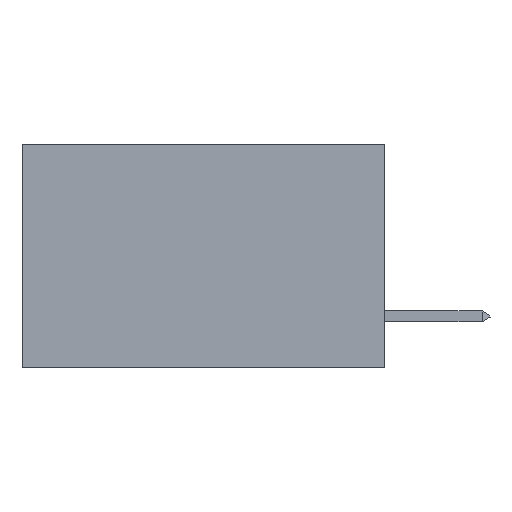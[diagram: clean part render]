
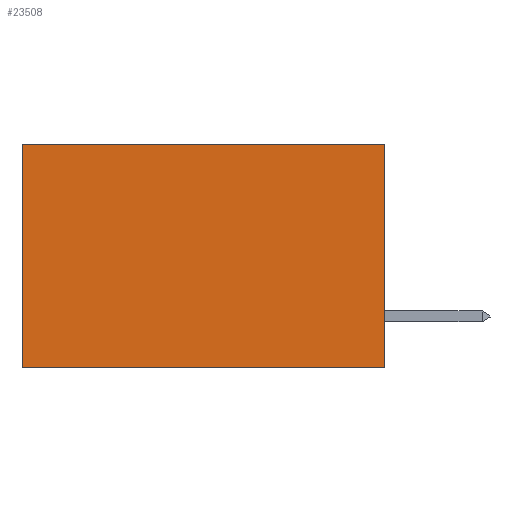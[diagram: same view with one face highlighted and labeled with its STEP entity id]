
A CAD part, left-side view. The second image highlights one B-rep face of the part: STEP entity #23508.
In plain terms, the highlighted planar face has unit normal (-1, 0, 0).
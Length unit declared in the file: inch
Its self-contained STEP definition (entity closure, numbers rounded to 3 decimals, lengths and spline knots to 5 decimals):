
#520 = ORIENTED_EDGE ( 'NONE', *, *, #11956, .F. ) ;
#1276 = EDGE_CURVE ( 'NONE', #7058, #15174, #4210, .T. ) ;
#1391 = ORIENTED_EDGE ( 'NONE', *, *, #22972, .F. ) ;
#1559 = CARTESIAN_POINT ( 'NONE',  ( 0.2875, 0., 0. ) ) ;
#1626 = VECTOR ( 'NONE', #16378, 39.37008 ) ;
#1716 = VECTOR ( 'NONE', #12483, 39.37008 ) ;
#3242 = CARTESIAN_POINT ( 'NONE',  ( 0.2875, 0., 0. ) ) ;
#3278 = DIRECTION ( 'NONE',  ( 0., 1., 0. ) ) ;
#3749 = LINE ( 'NONE', #4835, #1716 ) ;
#4210 = LINE ( 'NONE', #1559, #6255 ) ;
#4835 = CARTESIAN_POINT ( 'NONE',  ( 0.2875, 0.6, 0. ) ) ;
#6255 = VECTOR ( 'NONE', #3278, 39.37008 ) ;
#7043 = AXIS2_PLACEMENT_3D ( 'NONE', #15377, #22719, #13527 ) ;
#7058 = VERTEX_POINT ( 'NONE', #3242 ) ;
#7278 = VERTEX_POINT ( 'NONE', #19413 ) ;
#8296 = ORIENTED_EDGE ( 'NONE', *, *, #1276, .T. ) ;
#10164 = FACE_OUTER_BOUND ( 'NONE', #10364, .T. ) ;
#10183 = EDGE_CURVE ( 'NONE', #15174, #14729, #3749, .T. ) ;
#10364 = EDGE_LOOP ( 'NONE', ( #19242, #1391, #520, #8296 ) ) ;
#10704 = CARTESIAN_POINT ( 'NONE',  ( 0.2875, 0.6, -0.37 ) ) ;
#11956 = EDGE_CURVE ( 'NONE', #7058, #7278, #13223, .T. ) ;
#12483 = DIRECTION ( 'NONE',  ( 0., 0., -1. ) ) ;
#13223 = LINE ( 'NONE', #16225, #1626 ) ;
#13447 = PLANE ( 'NONE',  #7043 ) ;
#13527 = DIRECTION ( 'NONE',  ( 0., 0., -1. ) ) ;
#13793 = DIRECTION ( 'NONE',  ( 0., 1., 0. ) ) ;
#14729 = VERTEX_POINT ( 'NONE', #10704 ) ;
#15174 = VERTEX_POINT ( 'NONE', #18854 ) ;
#15377 = CARTESIAN_POINT ( 'NONE',  ( 0.2875, 0., 0. ) ) ;
#15714 = CARTESIAN_POINT ( 'NONE',  ( 0.2875, 0., -0.37 ) ) ;
#15948 = LINE ( 'NONE', #15714, #23793 ) ;
#16225 = CARTESIAN_POINT ( 'NONE',  ( 0.2875, 0., 0. ) ) ;
#16378 = DIRECTION ( 'NONE',  ( 0., 0., -1. ) ) ;
#18854 = CARTESIAN_POINT ( 'NONE',  ( 0.2875, 0.6, 0. ) ) ;
#19242 = ORIENTED_EDGE ( 'NONE', *, *, #10183, .T. ) ;
#19413 = CARTESIAN_POINT ( 'NONE',  ( 0.2875, 0., -0.37 ) ) ;
#22719 = DIRECTION ( 'NONE',  ( 1., 0., 0. ) ) ;
#22972 = EDGE_CURVE ( 'NONE', #7278, #14729, #15948, .T. ) ;
#23508 = ADVANCED_FACE ( 'NONE', ( #10164 ), #13447, .F. ) ;
#23793 = VECTOR ( 'NONE', #13793, 39.37008 ) ;
